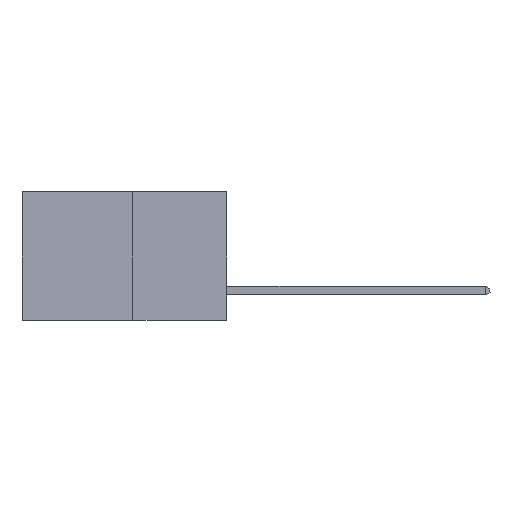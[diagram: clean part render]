
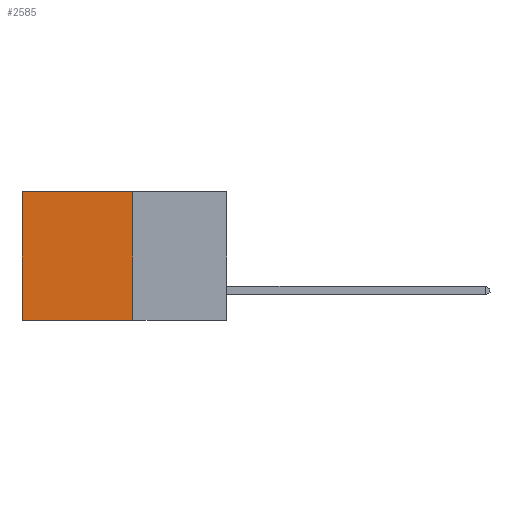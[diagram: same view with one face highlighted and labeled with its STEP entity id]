
A CAD part, left-side view. The second image highlights one B-rep face of the part: STEP entity #2585.
In plain terms, the highlighted planar face has unit normal (-1, 0, 0).
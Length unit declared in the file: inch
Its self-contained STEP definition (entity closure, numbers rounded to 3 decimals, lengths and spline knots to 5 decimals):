
#26 = EDGE_CURVE ( 'NONE', #1540, #11549, #4456, .T. ) ;
#68 = CARTESIAN_POINT ( 'NONE',  ( 0.277, 0.27, 0. ) ) ;
#312 = AXIS2_PLACEMENT_3D ( 'NONE', #9040, #4455, #12391 ) ;
#601 = LINE ( 'NONE', #8259, #6281 ) ;
#1139 = VECTOR ( 'NONE', #4683, 39.37008 ) ;
#1228 = ORIENTED_EDGE ( 'NONE', *, *, #13029, .F. ) ;
#1540 = VERTEX_POINT ( 'NONE', #2031 ) ;
#1959 = ORIENTED_EDGE ( 'NONE', *, *, #7484, .F. ) ;
#2031 = CARTESIAN_POINT ( 'NONE',  ( 0.277, 0.27, 0. ) ) ;
#2492 = CARTESIAN_POINT ( 'NONE',  ( 0.277, 0.59, -0.37 ) ) ;
#2585 = ADVANCED_FACE ( 'NONE', ( #8091 ), #13219, .F. ) ;
#2990 = LINE ( 'NONE', #5709, #11425 ) ;
#3222 = DIRECTION ( 'NONE',  ( 0., 0., -1. ) ) ;
#3456 = DIRECTION ( 'NONE',  ( 0., 1., 0. ) ) ;
#4067 = CARTESIAN_POINT ( 'NONE',  ( 0.277, 0.59, 0. ) ) ;
#4455 = DIRECTION ( 'NONE',  ( 1., 0., 0. ) ) ;
#4456 = LINE ( 'NONE', #68, #1139 ) ;
#4683 = DIRECTION ( 'NONE',  ( 0., 1., 0. ) ) ;
#5174 = LINE ( 'NONE', #2492, #13723 ) ;
#5253 = EDGE_LOOP ( 'NONE', ( #10027, #1228, #1959, #10076 ) ) ;
#5709 = CARTESIAN_POINT ( 'NONE',  ( 0.277, 0.27, -0.37 ) ) ;
#6281 = VECTOR ( 'NONE', #3222, 39.37008 ) ;
#7484 = EDGE_CURVE ( 'NONE', #1540, #14006, #601, .T. ) ;
#8091 = FACE_OUTER_BOUND ( 'NONE', #5253, .T. ) ;
#8259 = CARTESIAN_POINT ( 'NONE',  ( 0.277, 0.27, -0.37 ) ) ;
#9040 = CARTESIAN_POINT ( 'NONE',  ( 0.277, 0.27, -0.37 ) ) ;
#9425 = CARTESIAN_POINT ( 'NONE',  ( 0.277, 0.59, -0.37 ) ) ;
#10008 = EDGE_CURVE ( 'NONE', #11549, #11372, #5174, .T. ) ;
#10027 = ORIENTED_EDGE ( 'NONE', *, *, #10008, .T. ) ;
#10076 = ORIENTED_EDGE ( 'NONE', *, *, #26, .T. ) ;
#10188 = CARTESIAN_POINT ( 'NONE',  ( 0.277, 0.27, -0.37 ) ) ;
#11372 = VERTEX_POINT ( 'NONE', #9425 ) ;
#11425 = VECTOR ( 'NONE', #3456, 39.37008 ) ;
#11549 = VERTEX_POINT ( 'NONE', #4067 ) ;
#12287 = DIRECTION ( 'NONE',  ( 0., 0., -1. ) ) ;
#12391 = DIRECTION ( 'NONE',  ( 0., 0., -1. ) ) ;
#13029 = EDGE_CURVE ( 'NONE', #14006, #11372, #2990, .T. ) ;
#13219 = PLANE ( 'NONE',  #312 ) ;
#13723 = VECTOR ( 'NONE', #12287, 39.37008 ) ;
#14006 = VERTEX_POINT ( 'NONE', #10188 ) ;
